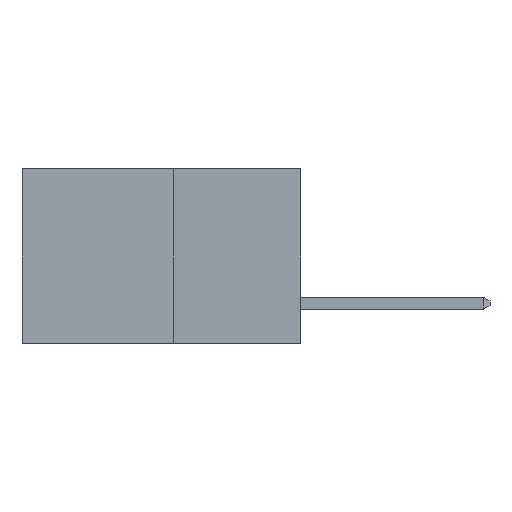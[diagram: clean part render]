
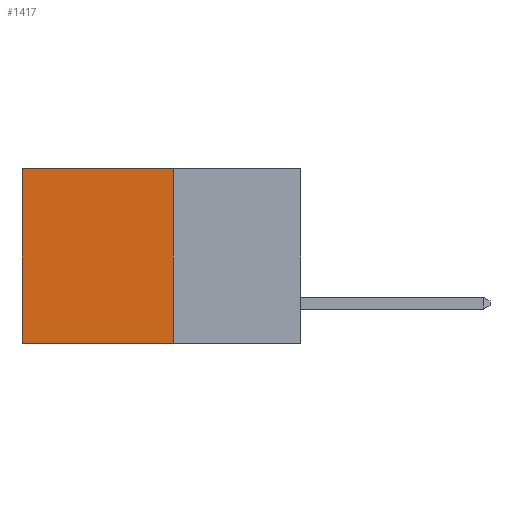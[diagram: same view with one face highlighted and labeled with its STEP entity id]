
A CAD part, left-side view. The second image highlights one B-rep face of the part: STEP entity #1417.
In plain terms, the highlighted planar face has unit normal (-1, 0, 0).
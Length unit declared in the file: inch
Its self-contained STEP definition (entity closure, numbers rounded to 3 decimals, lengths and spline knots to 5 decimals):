
#63 = VERTEX_POINT ( 'NONE', #4491 ) ;
#130 = CARTESIAN_POINT ( 'NONE',  ( 0.277, 0.27, -0.37 ) ) ;
#177 = DIRECTION ( 'NONE',  ( 0., 1., 0. ) ) ;
#187 = LINE ( 'NONE', #1242, #3593 ) ;
#687 = VERTEX_POINT ( 'NONE', #8325 ) ;
#793 = DIRECTION ( 'NONE',  ( 0., 0., -1. ) ) ;
#978 = VECTOR ( 'NONE', #7073, 39.37008 ) ;
#1242 = CARTESIAN_POINT ( 'NONE',  ( 0.277, 0.59, -0.37 ) ) ;
#1287 = ORIENTED_EDGE ( 'NONE', *, *, #3609, .T. ) ;
#1417 = ADVANCED_FACE ( 'NONE', ( #4660 ), #7603, .F. ) ;
#1736 = VECTOR ( 'NONE', #177, 39.37008 ) ;
#2099 = ORIENTED_EDGE ( 'NONE', *, *, #7248, .F. ) ;
#2385 = ORIENTED_EDGE ( 'NONE', *, *, #5277, .T. ) ;
#2387 = AXIS2_PLACEMENT_3D ( 'NONE', #7363, #7261, #7227 ) ;
#3353 = VERTEX_POINT ( 'NONE', #7150 ) ;
#3593 = VECTOR ( 'NONE', #793, 39.37008 ) ;
#3609 = EDGE_CURVE ( 'NONE', #63, #687, #187, .T. ) ;
#4491 = CARTESIAN_POINT ( 'NONE',  ( 0.277, 0.59, 0. ) ) ;
#4607 = VECTOR ( 'NONE', #7771, 39.37008 ) ;
#4660 = FACE_OUTER_BOUND ( 'NONE', #6021, .T. ) ;
#5163 = VERTEX_POINT ( 'NONE', #8153 ) ;
#5277 = EDGE_CURVE ( 'NONE', #5163, #63, #6252, .T. ) ;
#6021 = EDGE_LOOP ( 'NONE', ( #1287, #2099, #7567, #2385 ) ) ;
#6252 = LINE ( 'NONE', #7885, #4607 ) ;
#7032 = CARTESIAN_POINT ( 'NONE',  ( 0.277, 0.27, -0.37 ) ) ;
#7073 = DIRECTION ( 'NONE',  ( 0., 0., -1. ) ) ;
#7150 = CARTESIAN_POINT ( 'NONE',  ( 0.277, 0.27, -0.37 ) ) ;
#7227 = DIRECTION ( 'NONE',  ( 0., 0., -1. ) ) ;
#7248 = EDGE_CURVE ( 'NONE', #3353, #687, #8269, .T. ) ;
#7261 = DIRECTION ( 'NONE',  ( 1., 0., 0. ) ) ;
#7363 = CARTESIAN_POINT ( 'NONE',  ( 0.277, 0.27, -0.37 ) ) ;
#7567 = ORIENTED_EDGE ( 'NONE', *, *, #7978, .F. ) ;
#7592 = LINE ( 'NONE', #7032, #978 ) ;
#7603 = PLANE ( 'NONE',  #2387 ) ;
#7771 = DIRECTION ( 'NONE',  ( 0., 1., 0. ) ) ;
#7885 = CARTESIAN_POINT ( 'NONE',  ( 0.277, 0.27, 0. ) ) ;
#7978 = EDGE_CURVE ( 'NONE', #5163, #3353, #7592, .T. ) ;
#8153 = CARTESIAN_POINT ( 'NONE',  ( 0.277, 0.27, 0. ) ) ;
#8269 = LINE ( 'NONE', #130, #1736 ) ;
#8325 = CARTESIAN_POINT ( 'NONE',  ( 0.277, 0.59, -0.37 ) ) ;
